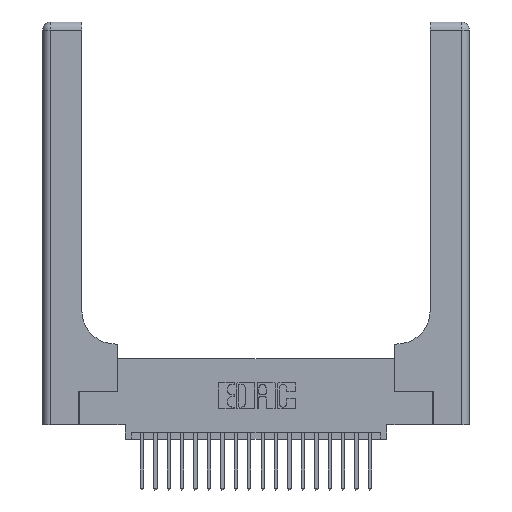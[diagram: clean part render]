
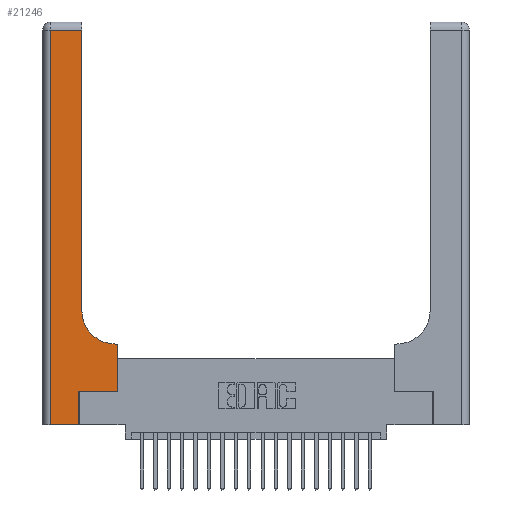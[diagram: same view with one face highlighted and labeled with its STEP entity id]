
A CAD part, top view. The second image highlights one B-rep face of the part: STEP entity #21246.
In plain terms, the highlighted planar face has unit normal (0, 0, 1).
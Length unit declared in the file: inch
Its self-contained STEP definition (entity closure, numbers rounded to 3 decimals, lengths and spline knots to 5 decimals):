
#189 = VERTEX_POINT ( 'NONE', #14032 ) ;
#377 = ORIENTED_EDGE ( 'NONE', *, *, #8570, .T. ) ;
#846 = LINE ( 'NONE', #21976, #4429 ) ;
#1836 = DIRECTION ( 'NONE',  ( 1., 0., 0. ) ) ;
#1872 = VECTOR ( 'NONE', #17014, 39.37008 ) ;
#2061 = DIRECTION ( 'NONE',  ( 0., 1., 0. ) ) ;
#2276 = DIRECTION ( 'NONE',  ( 0., 0., -1. ) ) ;
#2337 = VECTOR ( 'NONE', #6138, 39.37008 ) ;
#2379 = ORIENTED_EDGE ( 'NONE', *, *, #16596, .T. ) ;
#2818 = CARTESIAN_POINT ( 'NONE',  ( 0.5415, 0.6, 0.37 ) ) ;
#2965 = EDGE_CURVE ( 'NONE', #21245, #189, #8367, .T. ) ;
#3369 = VECTOR ( 'NONE', #17027, 39.37008 ) ;
#4176 = CARTESIAN_POINT ( 'NONE',  ( 0.269, 0., 0.37 ) ) ;
#4183 = LINE ( 'NONE', #20502, #15945 ) ;
#4291 = ORIENTED_EDGE ( 'NONE', *, *, #15364, .T. ) ;
#4429 = VECTOR ( 'NONE', #20526, 39.37008 ) ;
#4850 = ORIENTED_EDGE ( 'NONE', *, *, #22644, .T. ) ;
#5300 = CARTESIAN_POINT ( 'NONE',  ( 0., 0., 0.37 ) ) ;
#5396 = LINE ( 'NONE', #19354, #22675 ) ;
#5443 = CARTESIAN_POINT ( 'NONE',  ( 0.2915, 2.94, 0.37 ) ) ;
#5838 = ORIENTED_EDGE ( 'NONE', *, *, #2965, .T. ) ;
#6070 = EDGE_CURVE ( 'NONE', #19024, #22350, #4183, .T. ) ;
#6138 = DIRECTION ( 'NONE',  ( 0., 1., 0. ) ) ;
#6517 = CARTESIAN_POINT ( 'NONE',  ( 0., 2.94, 0.37 ) ) ;
#6541 = LINE ( 'NONE', #6517, #1872 ) ;
#6944 = LINE ( 'NONE', #8372, #3369 ) ;
#7550 = VECTOR ( 'NONE', #2061, 39.37008 ) ;
#7709 = CARTESIAN_POINT ( 'NONE',  ( 0., 3., 0.37 ) ) ;
#8367 = LINE ( 'NONE', #9647, #2337 ) ;
#8372 = CARTESIAN_POINT ( 'NONE',  ( 0.269, 0.25, 0.37 ) ) ;
#8391 = DIRECTION ( 'NONE',  ( 0., 1., 0. ) ) ;
#8513 = ORIENTED_EDGE ( 'NONE', *, *, #11635, .T. ) ;
#8570 = EDGE_CURVE ( 'NONE', #22350, #8688, #6541, .T. ) ;
#8688 = VERTEX_POINT ( 'NONE', #10043 ) ;
#9081 = AXIS2_PLACEMENT_3D ( 'NONE', #7709, #2276, #11238 ) ;
#9330 = PLANE ( 'NONE',  #9081 ) ;
#9647 = CARTESIAN_POINT ( 'NONE',  ( 0.269, 0., 0.37 ) ) ;
#9765 = ORIENTED_EDGE ( 'NONE', *, *, #6070, .T. ) ;
#10043 = CARTESIAN_POINT ( 'NONE',  ( 0.06, 2.94, 0.37 ) ) ;
#10094 = CARTESIAN_POINT ( 'NONE',  ( 0.5585, 0.25, 0.37 ) ) ;
#10537 = LINE ( 'NONE', #5300, #11640 ) ;
#11238 = DIRECTION ( 'NONE',  ( -1., 0., 0. ) ) ;
#11635 = EDGE_CURVE ( 'NONE', #16850, #19024, #14856, .T. ) ;
#11640 = VECTOR ( 'NONE', #12294, 39.37008 ) ;
#11812 = VERTEX_POINT ( 'NONE', #18807 ) ;
#12274 = CARTESIAN_POINT ( 'NONE',  ( 0.5415, 0.85, 0.37 ) ) ;
#12294 = DIRECTION ( 'NONE',  ( 1., 0., 0. ) ) ;
#12477 = FACE_OUTER_BOUND ( 'NONE', #15135, .T. ) ;
#13546 = ORIENTED_EDGE ( 'NONE', *, *, #21691, .T. ) ;
#14022 = DIRECTION ( 'NONE',  ( 0., 0., -1. ) ) ;
#14032 = CARTESIAN_POINT ( 'NONE',  ( 0.269, 0.25, 0.37 ) ) ;
#14191 = VERTEX_POINT ( 'NONE', #20027 ) ;
#14856 = CIRCLE ( 'NONE', #15227, 0.25 ) ;
#15135 = EDGE_LOOP ( 'NONE', ( #9765, #377, #4291, #13546, #5838, #21936, #2379, #4850, #8513 ) ) ;
#15227 = AXIS2_PLACEMENT_3D ( 'NONE', #12274, #14022, #1836 ) ;
#15364 = EDGE_CURVE ( 'NONE', #8688, #14191, #5396, .T. ) ;
#15945 = VECTOR ( 'NONE', #8391, 39.37008 ) ;
#15978 = DIRECTION ( 'NONE',  ( 0., -1., 0. ) ) ;
#16596 = EDGE_CURVE ( 'NONE', #16939, #11812, #16876, .T. ) ;
#16850 = VERTEX_POINT ( 'NONE', #2818 ) ;
#16876 = LINE ( 'NONE', #17467, #7550 ) ;
#16939 = VERTEX_POINT ( 'NONE', #10094 ) ;
#17014 = DIRECTION ( 'NONE',  ( -1., 0., 0. ) ) ;
#17027 = DIRECTION ( 'NONE',  ( 1., 0., 0. ) ) ;
#17467 = CARTESIAN_POINT ( 'NONE',  ( 0.5585, 0.25, 0.37 ) ) ;
#18807 = CARTESIAN_POINT ( 'NONE',  ( 0.5585, 0.6, 0.37 ) ) ;
#19024 = VERTEX_POINT ( 'NONE', #20072 ) ;
#19354 = CARTESIAN_POINT ( 'NONE',  ( 0.06, 3., 0.37 ) ) ;
#20027 = CARTESIAN_POINT ( 'NONE',  ( 0.06, 0., 0.37 ) ) ;
#20072 = CARTESIAN_POINT ( 'NONE',  ( 0.2915, 0.85, 0.37 ) ) ;
#20502 = CARTESIAN_POINT ( 'NONE',  ( 0.2915, 3., 0.37 ) ) ;
#20526 = DIRECTION ( 'NONE',  ( -1., 0., 0. ) ) ;
#21245 = VERTEX_POINT ( 'NONE', #4176 ) ;
#21246 = ADVANCED_FACE ( 'NONE', ( #12477 ), #9330, .F. ) ;
#21691 = EDGE_CURVE ( 'NONE', #14191, #21245, #10537, .T. ) ;
#21936 = ORIENTED_EDGE ( 'NONE', *, *, #22157, .T. ) ;
#21976 = CARTESIAN_POINT ( 'NONE',  ( 0.2915, 0.6, 0.37 ) ) ;
#22157 = EDGE_CURVE ( 'NONE', #189, #16939, #6944, .T. ) ;
#22350 = VERTEX_POINT ( 'NONE', #5443 ) ;
#22644 = EDGE_CURVE ( 'NONE', #11812, #16850, #846, .T. ) ;
#22675 = VECTOR ( 'NONE', #15978, 39.37008 ) ;
